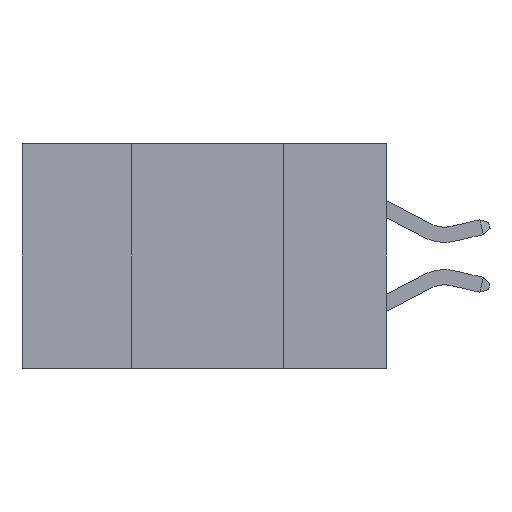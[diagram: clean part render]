
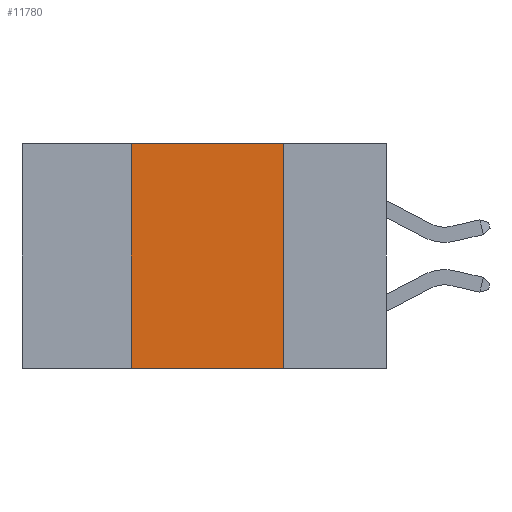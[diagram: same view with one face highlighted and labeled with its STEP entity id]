
A CAD part, left-side view. The second image highlights one B-rep face of the part: STEP entity #11780.
In plain terms, the highlighted planar face has unit normal (-1, 0, 0).
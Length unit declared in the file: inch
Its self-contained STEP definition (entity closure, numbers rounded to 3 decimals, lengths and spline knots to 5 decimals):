
#704 = FACE_OUTER_BOUND ( 'NONE', #1987, .T. ) ;
#925 = EDGE_CURVE ( 'NONE', #12241, #4859, #4408, .T. ) ;
#1289 = EDGE_CURVE ( 'NONE', #13689, #12241, #15017, .T. ) ;
#1411 = CARTESIAN_POINT ( 'NONE',  ( 0., 0.17, -0.37 ) ) ;
#1735 = ORIENTED_EDGE ( 'NONE', *, *, #925, .F. ) ;
#1987 = EDGE_LOOP ( 'NONE', ( #1735, #13158, #9495, #11801 ) ) ;
#2280 = CARTESIAN_POINT ( 'NONE',  ( 0., 0.42, -0.37 ) ) ;
#2433 = CARTESIAN_POINT ( 'NONE',  ( 0., 0.17, -0.37 ) ) ;
#3003 = CARTESIAN_POINT ( 'NONE',  ( 0., 0.42, 0. ) ) ;
#3475 = VECTOR ( 'NONE', #17887, 39.37008 ) ;
#3547 = DIRECTION ( 'NONE',  ( 0., 0., 1. ) ) ;
#3992 = DIRECTION ( 'NONE',  ( 1., 0., 0. ) ) ;
#4408 = LINE ( 'NONE', #1411, #17935 ) ;
#4859 = VERTEX_POINT ( 'NONE', #2433 ) ;
#5425 = DIRECTION ( 'NONE',  ( 0., 0., -1. ) ) ;
#6970 = CARTESIAN_POINT ( 'NONE',  ( 0., 0.6, 0. ) ) ;
#7460 = VECTOR ( 'NONE', #14805, 39.37008 ) ;
#9495 = ORIENTED_EDGE ( 'NONE', *, *, #19076, .F. ) ;
#10078 = CARTESIAN_POINT ( 'NONE',  ( 0., 0.6, 0. ) ) ;
#10236 = VERTEX_POINT ( 'NONE', #12398 ) ;
#11273 = EDGE_CURVE ( 'NONE', #10236, #4859, #15938, .T. ) ;
#11780 = ADVANCED_FACE ( 'NONE', ( #704 ), #19887, .F. ) ;
#11801 = ORIENTED_EDGE ( 'NONE', *, *, #11273, .T. ) ;
#12241 = VERTEX_POINT ( 'NONE', #18188 ) ;
#12398 = CARTESIAN_POINT ( 'NONE',  ( 0., 0.42, -0.37 ) ) ;
#13158 = ORIENTED_EDGE ( 'NONE', *, *, #1289, .F. ) ;
#13250 = CARTESIAN_POINT ( 'NONE',  ( 0., 0.6, -0.37 ) ) ;
#13689 = VERTEX_POINT ( 'NONE', #3003 ) ;
#13912 = AXIS2_PLACEMENT_3D ( 'NONE', #6970, #3992, #5425 ) ;
#14492 = LINE ( 'NONE', #2280, #15937 ) ;
#14805 = DIRECTION ( 'NONE',  ( 0., -1., 0. ) ) ;
#15017 = LINE ( 'NONE', #10078, #3475 ) ;
#15937 = VECTOR ( 'NONE', #3547, 39.37008 ) ;
#15938 = LINE ( 'NONE', #13250, #7460 ) ;
#16989 = DIRECTION ( 'NONE',  ( 0., 0., -1. ) ) ;
#17887 = DIRECTION ( 'NONE',  ( 0., -1., 0. ) ) ;
#17935 = VECTOR ( 'NONE', #16989, 39.37008 ) ;
#18188 = CARTESIAN_POINT ( 'NONE',  ( 0., 0.17, 0. ) ) ;
#19076 = EDGE_CURVE ( 'NONE', #10236, #13689, #14492, .T. ) ;
#19887 = PLANE ( 'NONE',  #13912 ) ;
